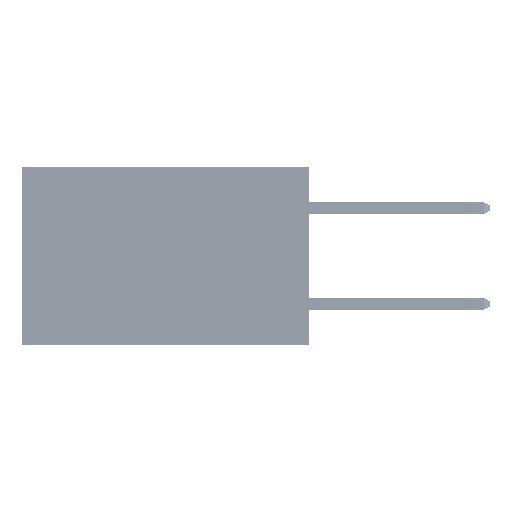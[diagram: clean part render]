
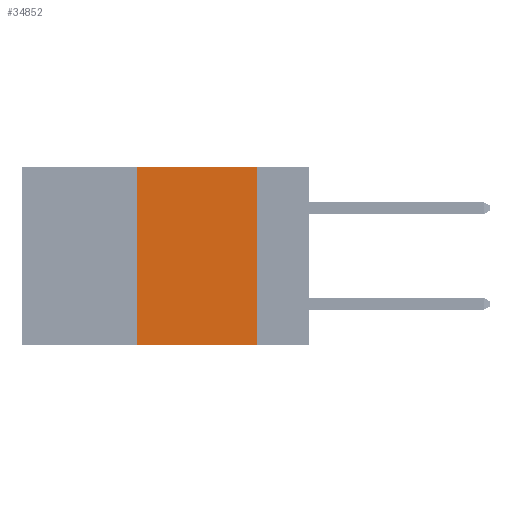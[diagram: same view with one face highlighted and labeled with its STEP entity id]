
A CAD part, left-side view. The second image highlights one B-rep face of the part: STEP entity #34852.
In plain terms, the highlighted planar face has unit normal (-1, 0, 0).
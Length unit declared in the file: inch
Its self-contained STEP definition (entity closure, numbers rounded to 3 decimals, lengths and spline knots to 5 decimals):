
#677 = CARTESIAN_POINT ( 'NONE',  ( 0., 0.6, 0. ) ) ;
#744 = LINE ( 'NONE', #42651, #10853 ) ;
#3317 = ORIENTED_EDGE ( 'NONE', *, *, #3606, .F. ) ;
#3606 = EDGE_CURVE ( 'NONE', #14414, #40229, #25946, .T. ) ;
#3836 = EDGE_CURVE ( 'NONE', #14414, #22697, #42648, .T. ) ;
#6018 = CARTESIAN_POINT ( 'NONE',  ( 0., 0.36, 0. ) ) ;
#7768 = FACE_OUTER_BOUND ( 'NONE', #13955, .T. ) ;
#8610 = VECTOR ( 'NONE', #43287, 39.37008 ) ;
#10166 = EDGE_CURVE ( 'NONE', #40229, #37606, #21025, .T. ) ;
#10627 = CARTESIAN_POINT ( 'NONE',  ( 0., 0.36, -0.37 ) ) ;
#10853 = VECTOR ( 'NONE', #39477, 39.37008 ) ;
#12243 = CARTESIAN_POINT ( 'NONE',  ( 0., 0.11, 0. ) ) ;
#13829 = DIRECTION ( 'NONE',  ( 0., -1., 0. ) ) ;
#13955 = EDGE_LOOP ( 'NONE', ( #40503, #21380, #3317, #20729 ) ) ;
#14166 = CARTESIAN_POINT ( 'NONE',  ( 0., 0.6, 0. ) ) ;
#14414 = VERTEX_POINT ( 'NONE', #10627 ) ;
#17209 = CARTESIAN_POINT ( 'NONE',  ( 0., 0.6, -0.37 ) ) ;
#17351 = DIRECTION ( 'NONE',  ( 0., 0., 1. ) ) ;
#19693 = AXIS2_PLACEMENT_3D ( 'NONE', #677, #31495, #42376 ) ;
#20141 = PLANE ( 'NONE',  #19693 ) ;
#20729 = ORIENTED_EDGE ( 'NONE', *, *, #3836, .T. ) ;
#21025 = LINE ( 'NONE', #14166, #25215 ) ;
#21380 = ORIENTED_EDGE ( 'NONE', *, *, #10166, .F. ) ;
#22697 = VERTEX_POINT ( 'NONE', #46759 ) ;
#22937 = VECTOR ( 'NONE', #17351, 39.37008 ) ;
#25215 = VECTOR ( 'NONE', #13829, 39.37008 ) ;
#25946 = LINE ( 'NONE', #6018, #22937 ) ;
#31495 = DIRECTION ( 'NONE',  ( 1., 0., 0. ) ) ;
#32425 = CARTESIAN_POINT ( 'NONE',  ( 0., 0.36, 0. ) ) ;
#33517 = EDGE_CURVE ( 'NONE', #37606, #22697, #744, .T. ) ;
#34852 = ADVANCED_FACE ( 'NONE', ( #7768 ), #20141, .F. ) ;
#37606 = VERTEX_POINT ( 'NONE', #12243 ) ;
#39477 = DIRECTION ( 'NONE',  ( 0., 0., -1. ) ) ;
#40229 = VERTEX_POINT ( 'NONE', #32425 ) ;
#40503 = ORIENTED_EDGE ( 'NONE', *, *, #33517, .F. ) ;
#42376 = DIRECTION ( 'NONE',  ( 0., 0., -1. ) ) ;
#42648 = LINE ( 'NONE', #17209, #8610 ) ;
#42651 = CARTESIAN_POINT ( 'NONE',  ( 0., 0.11, 0. ) ) ;
#43287 = DIRECTION ( 'NONE',  ( 0., -1., 0. ) ) ;
#46759 = CARTESIAN_POINT ( 'NONE',  ( 0., 0.11, -0.37 ) ) ;
